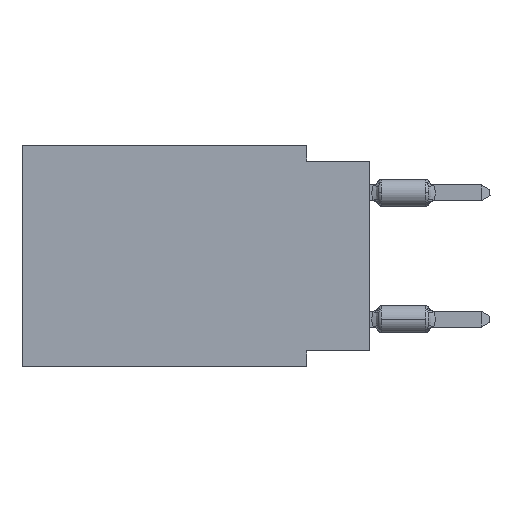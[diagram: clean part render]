
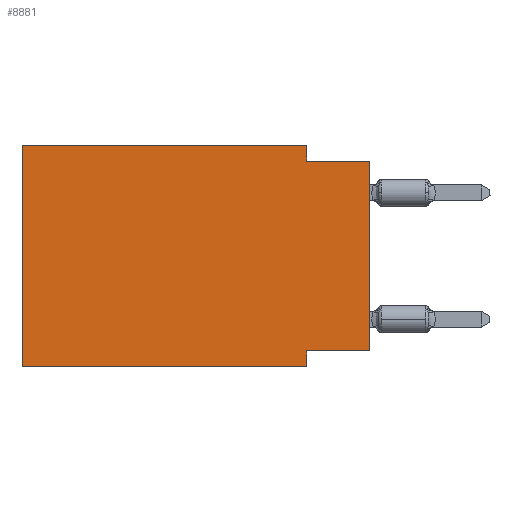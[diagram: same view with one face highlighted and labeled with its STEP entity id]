
A CAD part, left-side view. The second image highlights one B-rep face of the part: STEP entity #8881.
In plain terms, the highlighted planar face has unit normal (-1, 0, 0).
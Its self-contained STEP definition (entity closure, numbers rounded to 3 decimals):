
#240 = CARTESIAN_POINT ( 'NONE',  ( 0., 0., -8.255 ) ) ;
#1454 = VERTEX_POINT ( 'NONE', #48362 ) ;
#1833 = CARTESIAN_POINT ( 'NONE',  ( 0., 13.97, 0. ) ) ;
#2562 = LINE ( 'NONE', #16313, #19965 ) ;
#2930 = DIRECTION ( 'NONE',  ( 0., -1., 0. ) ) ;
#3002 = CARTESIAN_POINT ( 'NONE',  ( 0., 13.97, 0. ) ) ;
#3167 = ORIENTED_EDGE ( 'NONE', *, *, #34775, .T. ) ;
#3336 = VECTOR ( 'NONE', #54371, 1000. ) ;
#4270 = DIRECTION ( 'NONE',  ( 0., 1., 0. ) ) ;
#6152 = LINE ( 'NONE', #1833, #3336 ) ;
#6202 = DIRECTION ( 'NONE',  ( 0., 0., -1. ) ) ;
#8689 = ORIENTED_EDGE ( 'NONE', *, *, #17570, .F. ) ;
#8881 = ADVANCED_FACE ( 'NONE', ( #56678 ), #33711, .F. ) ;
#8916 = CARTESIAN_POINT ( 'NONE',  ( 0., 0., -8.255 ) ) ;
#10035 = LINE ( 'NONE', #41035, #27188 ) ;
#11319 = CARTESIAN_POINT ( 'NONE',  ( 0., 2.54, -8.89 ) ) ;
#12097 = LINE ( 'NONE', #50589, #52911 ) ;
#14630 = EDGE_CURVE ( 'NONE', #17639, #18497, #10035, .T. ) ;
#14659 = CARTESIAN_POINT ( 'NONE',  ( 0., 0., 0. ) ) ;
#16032 = EDGE_LOOP ( 'NONE', ( #56237, #24197, #53850, #32855, #32451, #3167, #8689, #42077 ) ) ;
#16313 = CARTESIAN_POINT ( 'NONE',  ( 0., 13.97, 0. ) ) ;
#16480 = DIRECTION ( 'NONE',  ( 0., 0., -1. ) ) ;
#17570 = EDGE_CURVE ( 'NONE', #47613, #28993, #28837, .T. ) ;
#17639 = VERTEX_POINT ( 'NONE', #19374 ) ;
#18497 = VERTEX_POINT ( 'NONE', #48130 ) ;
#18523 = VERTEX_POINT ( 'NONE', #39495 ) ;
#19374 = CARTESIAN_POINT ( 'NONE',  ( 0., 2.54, 0. ) ) ;
#19965 = VECTOR ( 'NONE', #38132, 1000. ) ;
#20662 = CARTESIAN_POINT ( 'NONE',  ( 0., 2.54, -8.255 ) ) ;
#24197 = ORIENTED_EDGE ( 'NONE', *, *, #50925, .F. ) ;
#24893 = DIRECTION ( 'NONE',  ( 0., 0., 1. ) ) ;
#25413 = LINE ( 'NONE', #34019, #26223 ) ;
#25514 = LINE ( 'NONE', #240, #28718 ) ;
#26223 = VECTOR ( 'NONE', #34307, 1000. ) ;
#27188 = VECTOR ( 'NONE', #40181, 1000. ) ;
#28718 = VECTOR ( 'NONE', #4270, 1000. ) ;
#28837 = LINE ( 'NONE', #11319, #51410 ) ;
#28993 = VERTEX_POINT ( 'NONE', #49503 ) ;
#32451 = ORIENTED_EDGE ( 'NONE', *, *, #35900, .F. ) ;
#32855 = ORIENTED_EDGE ( 'NONE', *, *, #56763, .F. ) ;
#33711 = PLANE ( 'NONE',  #43384 ) ;
#34019 = CARTESIAN_POINT ( 'NONE',  ( 0., 0., -0.635 ) ) ;
#34072 = LINE ( 'NONE', #14659, #53461 ) ;
#34307 = DIRECTION ( 'NONE',  ( 0., -1., 0. ) ) ;
#34775 = EDGE_CURVE ( 'NONE', #39822, #28993, #12097, .T. ) ;
#35900 = EDGE_CURVE ( 'NONE', #39822, #1454, #2562, .T. ) ;
#36897 = VERTEX_POINT ( 'NONE', #8916 ) ;
#38132 = DIRECTION ( 'NONE',  ( 0., 0., 1. ) ) ;
#39142 = DIRECTION ( 'NONE',  ( 1., 0., 0. ) ) ;
#39495 = CARTESIAN_POINT ( 'NONE',  ( 0., 0., -0.635 ) ) ;
#39822 = VERTEX_POINT ( 'NONE', #47242 ) ;
#40181 = DIRECTION ( 'NONE',  ( 0., 0., -1. ) ) ;
#41035 = CARTESIAN_POINT ( 'NONE',  ( 0., 2.54, 0. ) ) ;
#42077 = ORIENTED_EDGE ( 'NONE', *, *, #46400, .F. ) ;
#43384 = AXIS2_PLACEMENT_3D ( 'NONE', #3002, #39142, #16480 ) ;
#46400 = EDGE_CURVE ( 'NONE', #36897, #47613, #25514, .T. ) ;
#47242 = CARTESIAN_POINT ( 'NONE',  ( 0., 13.97, -8.89 ) ) ;
#47613 = VERTEX_POINT ( 'NONE', #20662 ) ;
#48130 = CARTESIAN_POINT ( 'NONE',  ( 0., 2.54, -0.635 ) ) ;
#48362 = CARTESIAN_POINT ( 'NONE',  ( 0., 13.97, 0. ) ) ;
#49503 = CARTESIAN_POINT ( 'NONE',  ( 0., 2.54, -8.89 ) ) ;
#50589 = CARTESIAN_POINT ( 'NONE',  ( 0., 13.97, -8.89 ) ) ;
#50925 = EDGE_CURVE ( 'NONE', #18497, #18523, #25413, .T. ) ;
#51410 = VECTOR ( 'NONE', #6202, 1000. ) ;
#52911 = VECTOR ( 'NONE', #2930, 1000. ) ;
#53461 = VECTOR ( 'NONE', #24893, 1000. ) ;
#53850 = ORIENTED_EDGE ( 'NONE', *, *, #14630, .F. ) ;
#54098 = EDGE_CURVE ( 'NONE', #36897, #18523, #34072, .T. ) ;
#54371 = DIRECTION ( 'NONE',  ( 0., -1., 0. ) ) ;
#56237 = ORIENTED_EDGE ( 'NONE', *, *, #54098, .T. ) ;
#56678 = FACE_OUTER_BOUND ( 'NONE', #16032, .T. ) ;
#56763 = EDGE_CURVE ( 'NONE', #1454, #17639, #6152, .T. ) ;
